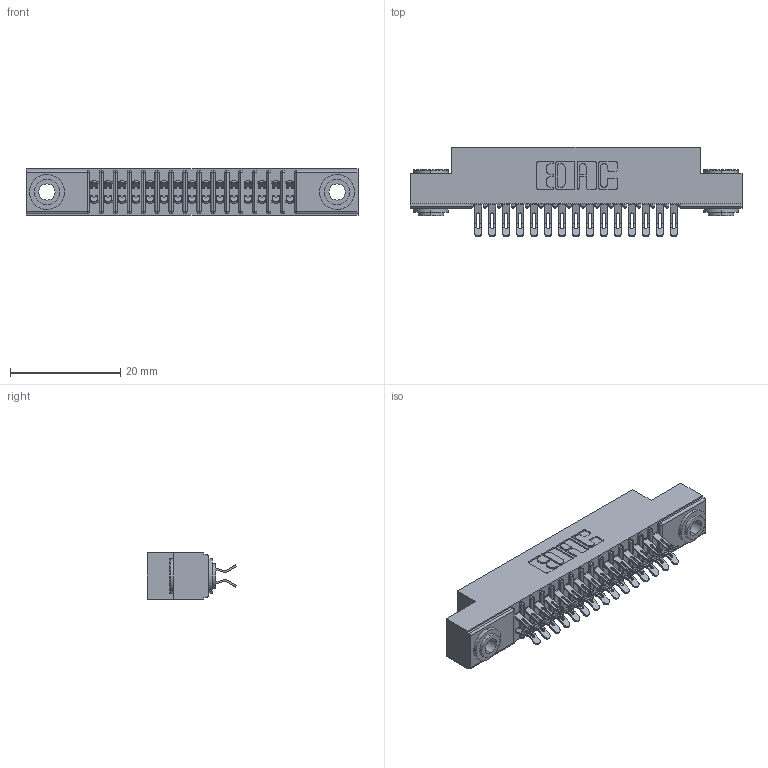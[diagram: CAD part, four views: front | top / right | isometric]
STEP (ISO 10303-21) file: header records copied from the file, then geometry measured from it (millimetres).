
FILE_DESCRIPTION (( 'STEP AP203' ), '1' );
FILE_NAME ('391-030-555-203.STEP', '2018-08-08T21:40:23', ( '' ), ( '' ), 'SwSTEP 2.0', 'SolidWorks 2016', '' );
FILE_SCHEMA (( 'CONFIG_CONTROL_DESIGN' ));
Length unit declared in the file: inch
Products named in the file (4): 341 Part_.156 (3.96) Dia Mounting Holes; 341-292-001_341-292-155; 345-250-002_345-250-002-102; 391-030-555-203
Assembly tree (33 placements, depth 2):
  391-030-555-203
    341 Part_.156 (3.96) Dia Mounting Holes
    341-292-001_341-292-155  x30
    345-250-002_345-250-002-102  x2
Bounding box: 60.33 x 16.31 x 8.38 mm (x, y, z)
Volume: 3492.9 mm3; surface area: 7320.9 mm2
Topology: 33 solids, 33 shells, 2508 faces, 7433 edges, 4838 vertices
Faces by surface type: plane 1352, cylinder 1088, sphere 32, torus 28, cone 8
Entity records: 23285 total; most frequent: CARTESIAN_POINT 3868, ORIENTED_EDGE 3822, DIRECTION 3779, EDGE_CURVE 1911, VECTOR 1489, LINE 1489, VERTEX_POINT 1218, AXIS2_PLACEMENT_3D 1145
